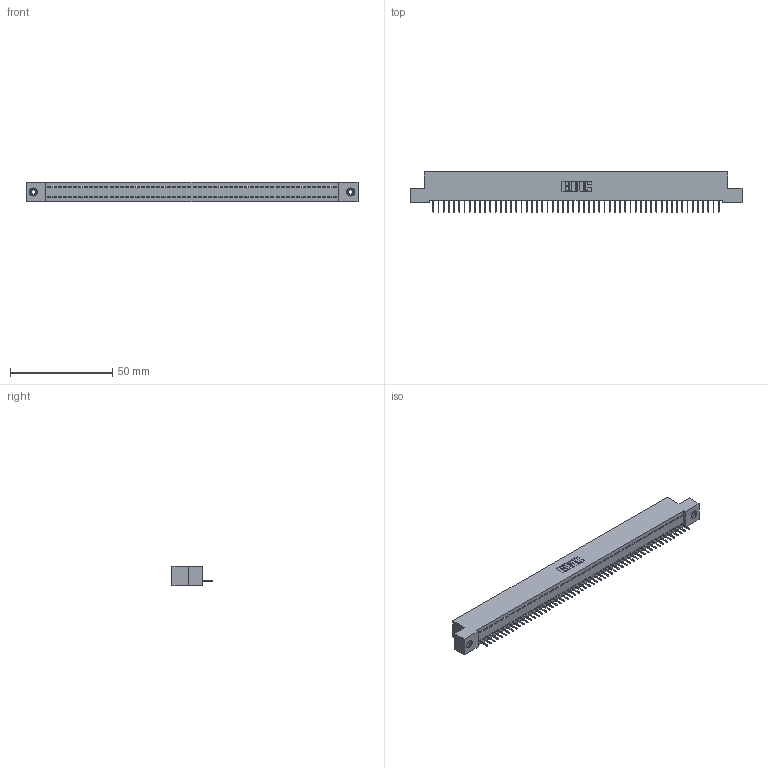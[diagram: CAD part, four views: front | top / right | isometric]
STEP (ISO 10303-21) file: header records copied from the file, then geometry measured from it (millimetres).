
FILE_DESCRIPTION (( 'STEP AP203' ), '1' );
FILE_NAME ('342-056-524-108.STEP', '2019-10-03T11:17:43', ( '' ), ( '' ), 'SwSTEP 2.0', 'SolidWorks 2016', '' );
FILE_SCHEMA (( 'CONFIG_CONTROL_DESIGN' ));
Length unit declared in the file: inch
Products named in the file (4): 342 Part_TI; 345-292-001_345-293-124; 345-250-001_345-250-003-102; 342-056-524-108
Assembly tree (59 placements, depth 2):
  342-056-524-108
    342 Part_TI
    345-292-001_345-293-124  x56
    345-250-001_345-250-003-102  x2
Bounding box: 162.56 x 19.69 x 9.4 mm (x, y, z)
Volume: 14077.9 mm3; surface area: 20264.9 mm2
Topology: 59 solids, 59 shells, 3642 faces, 10515 edges, 6778 vertices
Faces by surface type: plane 2786, cylinder 840, cone 12, torus 4
Entity records: 33552 total; most frequent: CARTESIAN_POINT 5765, ORIENTED_EDGE 5750, DIRECTION 4869, EDGE_CURVE 2875, VECTOR 2731, LINE 2731, VERTEX_POINT 1908, AXIS2_PLACEMENT_3D 1069
